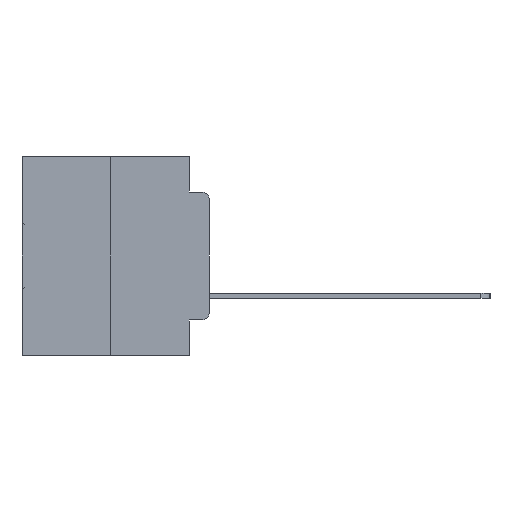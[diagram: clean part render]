
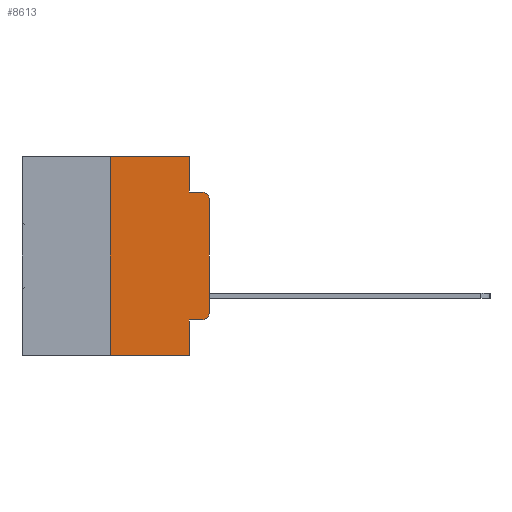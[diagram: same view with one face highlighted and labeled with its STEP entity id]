
A CAD part, left-side view. The second image highlights one B-rep face of the part: STEP entity #8613.
In plain terms, the highlighted planar face has unit normal (-1, 0, 0).
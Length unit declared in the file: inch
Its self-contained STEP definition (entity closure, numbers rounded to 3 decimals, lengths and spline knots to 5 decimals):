
#386 = EDGE_CURVE ( 'NONE', #21835, #8823, #30528, .T. ) ;
#912 = VERTEX_POINT ( 'NONE', #20072 ) ;
#1758 = CARTESIAN_POINT ( 'NONE',  ( 0., 0.051, -0.4115 ) ) ;
#1868 = VERTEX_POINT ( 'NONE', #29161 ) ;
#2423 = DIRECTION ( 'NONE',  ( 0., 0., -1. ) ) ;
#3113 = EDGE_CURVE ( 'NONE', #16220, #26770, #20988, .T. ) ;
#3121 = VECTOR ( 'NONE', #9384, 39.37008 ) ;
#4489 = AXIS2_PLACEMENT_3D ( 'NONE', #15059, #32524, #17587 ) ;
#4564 = CARTESIAN_POINT ( 'NONE',  ( 0., 0.051, -0.0885 ) ) ;
#4574 = DIRECTION ( 'NONE',  ( 0., 0., -1. ) ) ;
#5202 = CARTESIAN_POINT ( 'NONE',  ( 0., 0.02, -0.3915 ) ) ;
#6347 = CARTESIAN_POINT ( 'NONE',  ( 0., 0.051, 0. ) ) ;
#6842 = CIRCLE ( 'NONE', #23578, 0.02 ) ;
#6947 = EDGE_LOOP ( 'NONE', ( #16866, #16489, #27486, #26329, #16146, #26722, #25210, #20095, #32217, #25572 ) ) ;
#7489 = CARTESIAN_POINT ( 'NONE',  ( 0., 0.25, 0. ) ) ;
#7518 = VECTOR ( 'NONE', #11317, 39.37008 ) ;
#7822 = DIRECTION ( 'NONE',  ( 0., 0., -1. ) ) ;
#8613 = ADVANCED_FACE ( 'NONE', ( #24820 ), #11903, .F. ) ;
#8823 = VERTEX_POINT ( 'NONE', #17735 ) ;
#8859 = VECTOR ( 'NONE', #14059, 39.37008 ) ;
#9384 = DIRECTION ( 'NONE',  ( 0., -1., 0. ) ) ;
#9555 = VECTOR ( 'NONE', #29970, 39.37008 ) ;
#10076 = VECTOR ( 'NONE', #4574, 39.37008 ) ;
#10865 = LINE ( 'NONE', #32372, #10076 ) ;
#10892 = DIRECTION ( 'NONE',  ( 0., 0., 1. ) ) ;
#10954 = DIRECTION ( 'NONE',  ( 0., -1., 0. ) ) ;
#11317 = DIRECTION ( 'NONE',  ( 0., -1., 0. ) ) ;
#11619 = EDGE_CURVE ( 'NONE', #17805, #21835, #10865, .T. ) ;
#11903 = PLANE ( 'NONE',  #32625 ) ;
#12141 = EDGE_CURVE ( 'NONE', #31403, #1868, #22681, .T. ) ;
#12258 = CARTESIAN_POINT ( 'NONE',  ( 0., 0.25, -0.5 ) ) ;
#13285 = EDGE_CURVE ( 'NONE', #31403, #21368, #31993, .T. ) ;
#13377 = CARTESIAN_POINT ( 'NONE',  ( 0., 0.25, 0. ) ) ;
#14059 = DIRECTION ( 'NONE',  ( 0., -1., 0. ) ) ;
#14450 = CARTESIAN_POINT ( 'NONE',  ( 0., 0.473, 0. ) ) ;
#14532 = CARTESIAN_POINT ( 'NONE',  ( 0., 0.473, 0. ) ) ;
#15059 = CARTESIAN_POINT ( 'NONE',  ( 0., 0.02, -0.1085 ) ) ;
#16146 = ORIENTED_EDGE ( 'NONE', *, *, #26601, .F. ) ;
#16220 = VERTEX_POINT ( 'NONE', #1758 ) ;
#16329 = LINE ( 'NONE', #17267, #9555 ) ;
#16425 = VECTOR ( 'NONE', #2423, 39.37008 ) ;
#16489 = ORIENTED_EDGE ( 'NONE', *, *, #18618, .T. ) ;
#16866 = ORIENTED_EDGE ( 'NONE', *, *, #30367, .T. ) ;
#16965 = DIRECTION ( 'NONE',  ( 0., 0., -1. ) ) ;
#17170 = VERTEX_POINT ( 'NONE', #20881 ) ;
#17267 = CARTESIAN_POINT ( 'NONE',  ( 0., 0., 0. ) ) ;
#17587 = DIRECTION ( 'NONE',  ( 0., 0., -1. ) ) ;
#17735 = CARTESIAN_POINT ( 'NONE',  ( 0., 0.02, -0.0885 ) ) ;
#17805 = VERTEX_POINT ( 'NONE', #6347 ) ;
#18618 = EDGE_CURVE ( 'NONE', #912, #8823, #22905, .T. ) ;
#18705 = VECTOR ( 'NONE', #10892, 39.37008 ) ;
#18828 = CARTESIAN_POINT ( 'NONE',  ( 0., 0.051, -0.4115 ) ) ;
#19652 = CARTESIAN_POINT ( 'NONE',  ( 0., 0.051, -0.0885 ) ) ;
#20072 = CARTESIAN_POINT ( 'NONE',  ( 0., 0., -0.1085 ) ) ;
#20095 = ORIENTED_EDGE ( 'NONE', *, *, #29017, .F. ) ;
#20881 = CARTESIAN_POINT ( 'NONE',  ( 0., 0., -0.3915 ) ) ;
#20988 = LINE ( 'NONE', #18828, #7518 ) ;
#21368 = VERTEX_POINT ( 'NONE', #7489 ) ;
#21394 = EDGE_CURVE ( 'NONE', #26770, #17170, #6842, .T. ) ;
#21835 = VERTEX_POINT ( 'NONE', #19652 ) ;
#22627 = LINE ( 'NONE', #14532, #3121 ) ;
#22681 = LINE ( 'NONE', #26051, #27753 ) ;
#22905 = CIRCLE ( 'NONE', #4489, 0.02 ) ;
#22986 = DIRECTION ( 'NONE',  ( -1., 0., 0. ) ) ;
#23109 = LINE ( 'NONE', #32691, #16425 ) ;
#23578 = AXIS2_PLACEMENT_3D ( 'NONE', #5202, #22986, #7822 ) ;
#24820 = FACE_OUTER_BOUND ( 'NONE', #6947, .T. ) ;
#25158 = CARTESIAN_POINT ( 'NONE',  ( 0., 0.02, -0.4115 ) ) ;
#25210 = ORIENTED_EDGE ( 'NONE', *, *, #12141, .T. ) ;
#25572 = ORIENTED_EDGE ( 'NONE', *, *, #21394, .T. ) ;
#26051 = CARTESIAN_POINT ( 'NONE',  ( 0., 0.473, -0.5 ) ) ;
#26329 = ORIENTED_EDGE ( 'NONE', *, *, #11619, .F. ) ;
#26601 = EDGE_CURVE ( 'NONE', #21368, #17805, #22627, .T. ) ;
#26722 = ORIENTED_EDGE ( 'NONE', *, *, #13285, .F. ) ;
#26770 = VERTEX_POINT ( 'NONE', #25158 ) ;
#27486 = ORIENTED_EDGE ( 'NONE', *, *, #386, .F. ) ;
#27753 = VECTOR ( 'NONE', #10954, 39.37008 ) ;
#29017 = EDGE_CURVE ( 'NONE', #16220, #1868, #23109, .T. ) ;
#29161 = CARTESIAN_POINT ( 'NONE',  ( 0., 0.051, -0.5 ) ) ;
#29970 = DIRECTION ( 'NONE',  ( 0., 0., 1. ) ) ;
#30367 = EDGE_CURVE ( 'NONE', #17170, #912, #16329, .T. ) ;
#30528 = LINE ( 'NONE', #4564, #8859 ) ;
#31403 = VERTEX_POINT ( 'NONE', #12258 ) ;
#31925 = DIRECTION ( 'NONE',  ( 1., 0., 0. ) ) ;
#31993 = LINE ( 'NONE', #13377, #18705 ) ;
#32217 = ORIENTED_EDGE ( 'NONE', *, *, #3113, .T. ) ;
#32372 = CARTESIAN_POINT ( 'NONE',  ( 0., 0.051, 0. ) ) ;
#32524 = DIRECTION ( 'NONE',  ( -1., 0., 0. ) ) ;
#32625 = AXIS2_PLACEMENT_3D ( 'NONE', #14450, #31925, #16965 ) ;
#32691 = CARTESIAN_POINT ( 'NONE',  ( 0., 0.051, 0. ) ) ;
